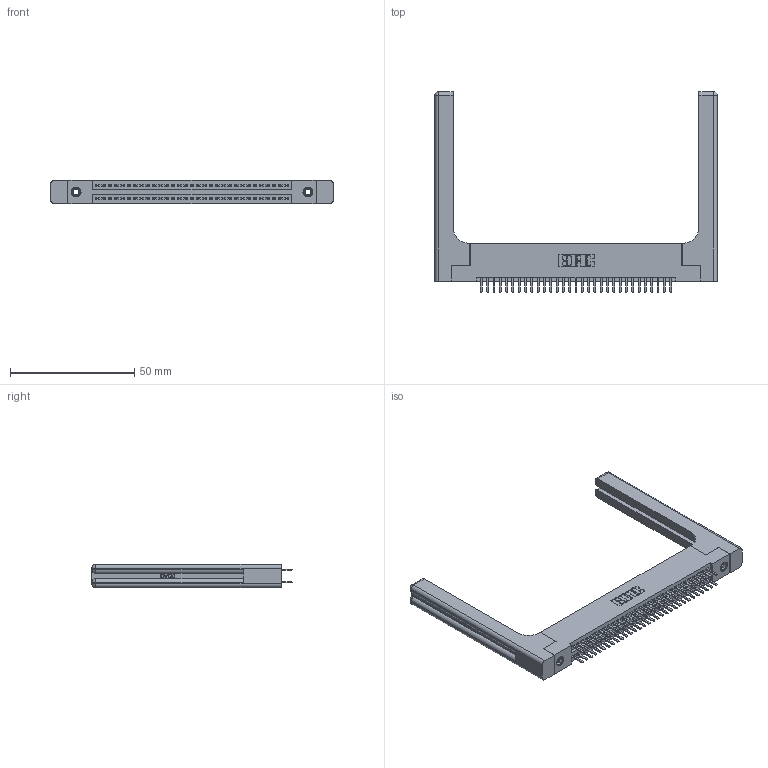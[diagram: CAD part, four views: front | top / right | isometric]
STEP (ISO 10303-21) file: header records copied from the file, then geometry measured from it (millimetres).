
FILE_DESCRIPTION (( 'STEP AP203' ), '1' );
FILE_NAME ('395-062-520-258.STEP', '2019-10-23T15:21:06', ( '' ), ( '' ), 'SwSTEP 2.0', 'SolidWorks 2016', '' );
FILE_SCHEMA (( 'CONFIG_CONTROL_DESIGN' ));
Length unit declared in the file: inch
Products named in the file (5): 345 Part_Flush Mounting Lugs - 0.156 Dia-TH; 345-292-001_345-293-120; 345-250-001_345-250-001-102; 345-220-058_345-220-058; 395-062-520-258
Assembly tree (67 placements, depth 2):
  395-062-520-258
    345 Part_Flush Mounting Lugs - 0.156 Dia-TH
    345-292-001_345-293-120  x62
    345-250-001_345-250-001-102  x2
    345-220-058_345-220-058  x2
Bounding box: 113.77 x 80.64 x 9.4 mm (x, y, z)
Volume: 19397.2 mm3; surface area: 20932.5 mm2
Topology: 67 solids, 67 shells, 3730 faces, 10741 edges, 6974 vertices
Faces by surface type: plane 2398, cylinder 1272, bspline 36, cone 12, sphere 8, torus 4
Entity records: 31100 total; most frequent: CARTESIAN_POINT 6229, ORIENTED_EDGE 4948, DIRECTION 4426, EDGE_CURVE 2474, LINE 2122, VECTOR 2122, VERTEX_POINT 1638, AXIS2_PLACEMENT_3D 1152
